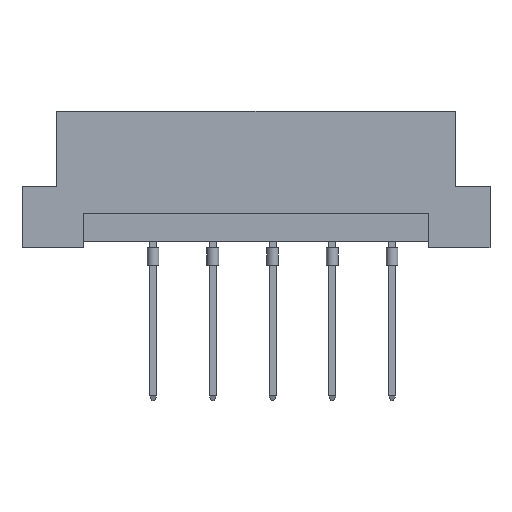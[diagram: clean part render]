
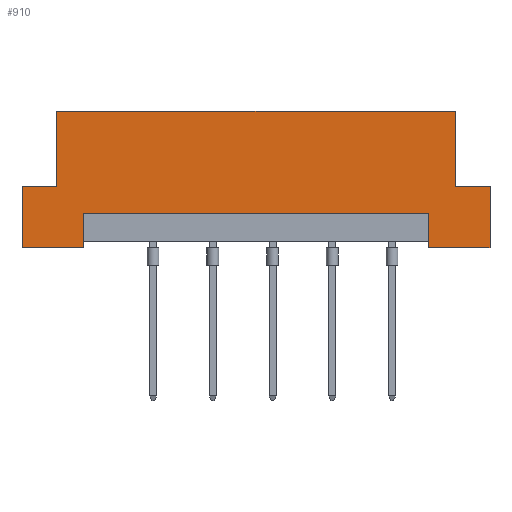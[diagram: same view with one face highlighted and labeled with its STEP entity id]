
A CAD part, front view. The second image highlights one B-rep face of the part: STEP entity #910.
In plain terms, the highlighted planar face has unit normal (0, -1, 0).
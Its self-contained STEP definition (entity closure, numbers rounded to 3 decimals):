
#10 = CARTESIAN_POINT ( 'NONE',  ( -19.9, 0., 11.6 ) ) ;
#35 = LINE ( 'NONE', #6434, #2371 ) ;
#38 = EDGE_CURVE ( 'NONE', #3510, #3752, #2030, .T. ) ;
#82 = CARTESIAN_POINT ( 'NONE',  ( 14.69, 0., 0. ) ) ;
#112 = DIRECTION ( 'NONE',  ( 0., 0., -1. ) ) ;
#231 = VECTOR ( 'NONE', #2421, 1000. ) ;
#393 = VECTOR ( 'NONE', #5490, 1000. ) ;
#469 = EDGE_CURVE ( 'NONE', #1661, #3510, #3750, .T. ) ;
#606 = LINE ( 'NONE', #6475, #6806 ) ;
#802 = LINE ( 'NONE', #3865, #1784 ) ;
#829 = EDGE_CURVE ( 'NONE', #4201, #4979, #1914, .T. ) ;
#910 = ADVANCED_FACE ( 'NONE', ( #6335 ), #2656, .F. ) ;
#1237 = ORIENTED_EDGE ( 'NONE', *, *, #38, .F. ) ;
#1398 = ORIENTED_EDGE ( 'NONE', *, *, #2761, .F. ) ;
#1520 = CARTESIAN_POINT ( 'NONE',  ( -16.94, 0., 5.2 ) ) ;
#1587 = EDGE_CURVE ( 'NONE', #4355, #4677, #5558, .T. ) ;
#1622 = CARTESIAN_POINT ( 'NONE',  ( -19.9, 0., 11.6 ) ) ;
#1661 = VERTEX_POINT ( 'NONE', #5591 ) ;
#1784 = VECTOR ( 'NONE', #5001, 1000. ) ;
#1788 = DIRECTION ( 'NONE',  ( -1., 0., 0. ) ) ;
#1826 = ORIENTED_EDGE ( 'NONE', *, *, #5399, .F. ) ;
#1864 = CARTESIAN_POINT ( 'NONE',  ( 16.94, 0., 5.2 ) ) ;
#1914 = LINE ( 'NONE', #4492, #4112 ) ;
#1974 = CARTESIAN_POINT ( 'NONE',  ( 14.69, 0., 2.9 ) ) ;
#2015 = EDGE_CURVE ( 'NONE', #4206, #5876, #802, .T. ) ;
#2030 = LINE ( 'NONE', #6753, #3478 ) ;
#2032 = LINE ( 'NONE', #2496, #6858 ) ;
#2123 = EDGE_LOOP ( 'NONE', ( #3178, #2526, #1398, #2775, #4912, #4562, #3369, #3259, #3421, #1237, #3383, #1826 ) ) ;
#2296 = VECTOR ( 'NONE', #3744, 1000. ) ;
#2358 = VERTEX_POINT ( 'NONE', #82 ) ;
#2371 = VECTOR ( 'NONE', #4972, 1000. ) ;
#2400 = VECTOR ( 'NONE', #4004, 1000. ) ;
#2421 = DIRECTION ( 'NONE',  ( 0., 0., 1. ) ) ;
#2496 = CARTESIAN_POINT ( 'NONE',  ( 14.69, 0., 0.5 ) ) ;
#2526 = ORIENTED_EDGE ( 'NONE', *, *, #3531, .T. ) ;
#2541 = LINE ( 'NONE', #1864, #393 ) ;
#2581 = VECTOR ( 'NONE', #1788, 1000. ) ;
#2619 = CARTESIAN_POINT ( 'NONE',  ( -19.9, 0., 0. ) ) ;
#2656 = PLANE ( 'NONE',  #3347 ) ;
#2761 = EDGE_CURVE ( 'NONE', #4033, #2358, #5452, .T. ) ;
#2775 = ORIENTED_EDGE ( 'NONE', *, *, #3245, .F. ) ;
#2825 = EDGE_CURVE ( 'NONE', #3752, #4355, #35, .T. ) ;
#2956 = CARTESIAN_POINT ( 'NONE',  ( 19.9, 0., 5.2 ) ) ;
#2975 = LINE ( 'NONE', #3387, #2400 ) ;
#3051 = CARTESIAN_POINT ( 'NONE',  ( -16.94, 0., 11.6 ) ) ;
#3054 = DIRECTION ( 'NONE',  ( 0., 0., 1. ) ) ;
#3178 = ORIENTED_EDGE ( 'NONE', *, *, #829, .F. ) ;
#3245 = EDGE_CURVE ( 'NONE', #5876, #4033, #606, .T. ) ;
#3259 = ORIENTED_EDGE ( 'NONE', *, *, #1587, .F. ) ;
#3316 = EDGE_CURVE ( 'NONE', #4677, #6626, #3323, .T. ) ;
#3323 = LINE ( 'NONE', #1622, #2296 ) ;
#3347 = AXIS2_PLACEMENT_3D ( 'NONE', #10, #6274, #3054 ) ;
#3369 = ORIENTED_EDGE ( 'NONE', *, *, #3316, .F. ) ;
#3383 = ORIENTED_EDGE ( 'NONE', *, *, #469, .F. ) ;
#3387 = CARTESIAN_POINT ( 'NONE',  ( -14.69, 0., 0.5 ) ) ;
#3421 = ORIENTED_EDGE ( 'NONE', *, *, #2825, .F. ) ;
#3478 = VECTOR ( 'NONE', #4689, 1000. ) ;
#3510 = VERTEX_POINT ( 'NONE', #2619 ) ;
#3531 = EDGE_CURVE ( 'NONE', #4201, #2358, #2032, .T. ) ;
#3744 = DIRECTION ( 'NONE',  ( 1., 0., 0. ) ) ;
#3750 = LINE ( 'NONE', #6379, #5158 ) ;
#3752 = VERTEX_POINT ( 'NONE', #5078 ) ;
#3823 = CARTESIAN_POINT ( 'NONE',  ( 19.9, 0., 0. ) ) ;
#3865 = CARTESIAN_POINT ( 'NONE',  ( 19.9, 0., 5.2 ) ) ;
#3875 = EDGE_CURVE ( 'NONE', #4206, #6626, #2541, .T. ) ;
#4004 = DIRECTION ( 'NONE',  ( 0., 0., -1. ) ) ;
#4033 = VERTEX_POINT ( 'NONE', #3823 ) ;
#4094 = CARTESIAN_POINT ( 'NONE',  ( 16.94, 0., 5.2 ) ) ;
#4112 = VECTOR ( 'NONE', #6629, 1000. ) ;
#4200 = DIRECTION ( 'NONE',  ( -1., 0., 0. ) ) ;
#4201 = VERTEX_POINT ( 'NONE', #1974 ) ;
#4206 = VERTEX_POINT ( 'NONE', #4094 ) ;
#4355 = VERTEX_POINT ( 'NONE', #1520 ) ;
#4492 = CARTESIAN_POINT ( 'NONE',  ( 14.69, 0., 2.9 ) ) ;
#4510 = CARTESIAN_POINT ( 'NONE',  ( -16.94, 0., 5.2 ) ) ;
#4562 = ORIENTED_EDGE ( 'NONE', *, *, #3875, .T. ) ;
#4631 = DIRECTION ( 'NONE',  ( 0., 0., -1. ) ) ;
#4677 = VERTEX_POINT ( 'NONE', #3051 ) ;
#4689 = DIRECTION ( 'NONE',  ( 0., 0., 1. ) ) ;
#4901 = CARTESIAN_POINT ( 'NONE',  ( -19.9, 0., 0. ) ) ;
#4912 = ORIENTED_EDGE ( 'NONE', *, *, #2015, .F. ) ;
#4972 = DIRECTION ( 'NONE',  ( 1., 0., 0. ) ) ;
#4979 = VERTEX_POINT ( 'NONE', #5594 ) ;
#5001 = DIRECTION ( 'NONE',  ( 1., 0., 0. ) ) ;
#5078 = CARTESIAN_POINT ( 'NONE',  ( -19.9, 0., 5.2 ) ) ;
#5158 = VECTOR ( 'NONE', #4200, 1000. ) ;
#5399 = EDGE_CURVE ( 'NONE', #4979, #1661, #2975, .T. ) ;
#5452 = LINE ( 'NONE', #4901, #2581 ) ;
#5490 = DIRECTION ( 'NONE',  ( 0., 0., 1. ) ) ;
#5558 = LINE ( 'NONE', #4510, #231 ) ;
#5591 = CARTESIAN_POINT ( 'NONE',  ( -14.69, 0., 0. ) ) ;
#5594 = CARTESIAN_POINT ( 'NONE',  ( -14.69, 0., 2.9 ) ) ;
#5876 = VERTEX_POINT ( 'NONE', #2956 ) ;
#6274 = DIRECTION ( 'NONE',  ( 0., 1., 0. ) ) ;
#6335 = FACE_OUTER_BOUND ( 'NONE', #2123, .T. ) ;
#6379 = CARTESIAN_POINT ( 'NONE',  ( -19.9, 0., 0. ) ) ;
#6434 = CARTESIAN_POINT ( 'NONE',  ( -19.9, 0., 5.2 ) ) ;
#6461 = CARTESIAN_POINT ( 'NONE',  ( 16.94, 0., 11.6 ) ) ;
#6475 = CARTESIAN_POINT ( 'NONE',  ( 19.9, 0., 0. ) ) ;
#6626 = VERTEX_POINT ( 'NONE', #6461 ) ;
#6629 = DIRECTION ( 'NONE',  ( -1., 0., 0. ) ) ;
#6753 = CARTESIAN_POINT ( 'NONE',  ( -19.9, 0., 0. ) ) ;
#6806 = VECTOR ( 'NONE', #112, 1000. ) ;
#6858 = VECTOR ( 'NONE', #4631, 1000. ) ;
